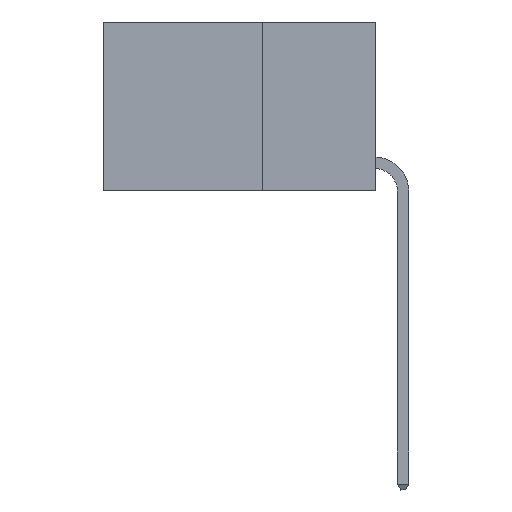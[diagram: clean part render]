
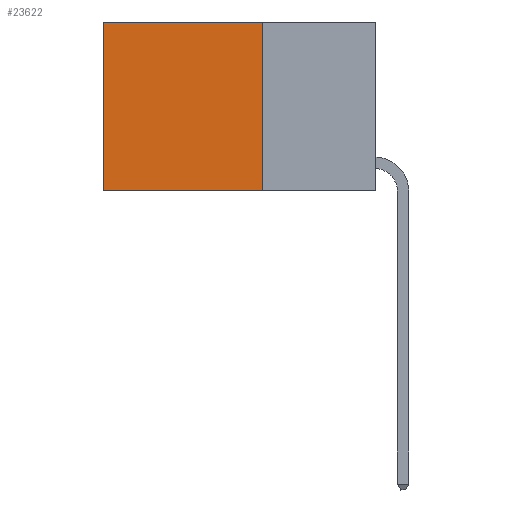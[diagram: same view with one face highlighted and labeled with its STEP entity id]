
A CAD part, left-side view. The second image highlights one B-rep face of the part: STEP entity #23622.
In plain terms, the highlighted planar face has unit normal (-1, 0, 0).
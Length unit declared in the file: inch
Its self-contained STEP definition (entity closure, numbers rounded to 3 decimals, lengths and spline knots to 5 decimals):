
#1041 = EDGE_LOOP ( 'NONE', ( #24968, #9632, #13447, #9627 ) ) ;
#2315 = FACE_OUTER_BOUND ( 'NONE', #1041, .T. ) ;
#3546 = CARTESIAN_POINT ( 'NONE',  ( 0.2625, 0.25, 0. ) ) ;
#3580 = LINE ( 'NONE', #8126, #22716 ) ;
#4960 = VECTOR ( 'NONE', #11948, 39.37008 ) ;
#5416 = EDGE_CURVE ( 'NONE', #11334, #13880, #9918, .T. ) ;
#6417 = DIRECTION ( 'NONE',  ( 0., 0., -1. ) ) ;
#6498 = VECTOR ( 'NONE', #16583, 39.37008 ) ;
#6565 = DIRECTION ( 'NONE',  ( 1., 0., 0. ) ) ;
#6730 = LINE ( 'NONE', #27901, #12275 ) ;
#7655 = VERTEX_POINT ( 'NONE', #21483 ) ;
#8126 = CARTESIAN_POINT ( 'NONE',  ( 0.2625, 0.25, 0. ) ) ;
#9116 = AXIS2_PLACEMENT_3D ( 'NONE', #25891, #6565, #6417 ) ;
#9627 = ORIENTED_EDGE ( 'NONE', *, *, #26060, .T. ) ;
#9632 = ORIENTED_EDGE ( 'NONE', *, *, #5416, .F. ) ;
#9918 = LINE ( 'NONE', #16039, #6498 ) ;
#11334 = VERTEX_POINT ( 'NONE', #20763 ) ;
#11948 = DIRECTION ( 'NONE',  ( 0., 0., -1. ) ) ;
#12275 = VECTOR ( 'NONE', #21629, 39.37008 ) ;
#13447 = ORIENTED_EDGE ( 'NONE', *, *, #20215, .F. ) ;
#13880 = VERTEX_POINT ( 'NONE', #19961 ) ;
#16039 = CARTESIAN_POINT ( 'NONE',  ( 0.2625, 0.25, -0.37 ) ) ;
#16583 = DIRECTION ( 'NONE',  ( 0., 1., 0. ) ) ;
#19196 = DIRECTION ( 'NONE',  ( 0., 1., 0. ) ) ;
#19961 = CARTESIAN_POINT ( 'NONE',  ( 0.2625, 0.6, -0.37 ) ) ;
#20215 = EDGE_CURVE ( 'NONE', #26553, #11334, #22736, .T. ) ;
#20763 = CARTESIAN_POINT ( 'NONE',  ( 0.2625, 0.25, -0.37 ) ) ;
#21483 = CARTESIAN_POINT ( 'NONE',  ( 0.2625, 0.6, 0. ) ) ;
#21629 = DIRECTION ( 'NONE',  ( 0., 0., -1. ) ) ;
#21975 = EDGE_CURVE ( 'NONE', #7655, #13880, #6730, .T. ) ;
#22716 = VECTOR ( 'NONE', #19196, 39.37008 ) ;
#22736 = LINE ( 'NONE', #27442, #4960 ) ;
#23622 = ADVANCED_FACE ( 'NONE', ( #2315 ), #25752, .F. ) ;
#24968 = ORIENTED_EDGE ( 'NONE', *, *, #21975, .T. ) ;
#25752 = PLANE ( 'NONE',  #9116 ) ;
#25891 = CARTESIAN_POINT ( 'NONE',  ( 0.2625, 0.25, 0. ) ) ;
#26060 = EDGE_CURVE ( 'NONE', #26553, #7655, #3580, .T. ) ;
#26553 = VERTEX_POINT ( 'NONE', #3546 ) ;
#27442 = CARTESIAN_POINT ( 'NONE',  ( 0.2625, 0.25, 0. ) ) ;
#27901 = CARTESIAN_POINT ( 'NONE',  ( 0.2625, 0.6, 0. ) ) ;
